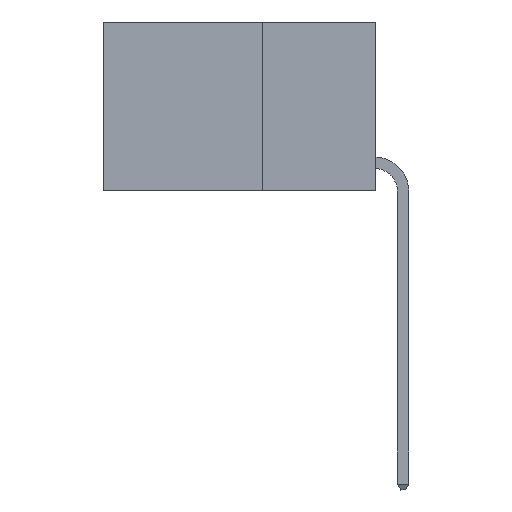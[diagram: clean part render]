
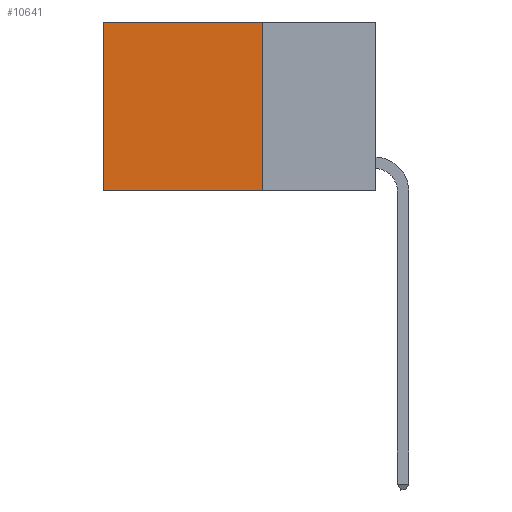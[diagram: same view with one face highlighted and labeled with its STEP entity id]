
A CAD part, left-side view. The second image highlights one B-rep face of the part: STEP entity #10641.
In plain terms, the highlighted planar face has unit normal (-1, 0, 0).
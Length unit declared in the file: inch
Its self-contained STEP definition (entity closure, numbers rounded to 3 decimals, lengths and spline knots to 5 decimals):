
#383 = ORIENTED_EDGE ( 'NONE', *, *, #12146, .T. ) ;
#412 = LINE ( 'NONE', #11326, #17715 ) ;
#622 = EDGE_CURVE ( 'NONE', #13639, #8643, #17457, .T. ) ;
#641 = CARTESIAN_POINT ( 'NONE',  ( 0.2625, 0.25, 0. ) ) ;
#673 = CARTESIAN_POINT ( 'NONE',  ( 0.2625, 0.6, 0. ) ) ;
#1697 = LINE ( 'NONE', #18123, #5662 ) ;
#2120 = DIRECTION ( 'NONE',  ( 0., 1., 0. ) ) ;
#2247 = DIRECTION ( 'NONE',  ( 0., 1., 0. ) ) ;
#3027 = VERTEX_POINT ( 'NONE', #14223 ) ;
#3090 = FACE_OUTER_BOUND ( 'NONE', #8799, .T. ) ;
#4413 = PLANE ( 'NONE',  #12980 ) ;
#5662 = VECTOR ( 'NONE', #7808, 39.37008 ) ;
#5687 = DIRECTION ( 'NONE',  ( 0., 0., -1. ) ) ;
#5933 = EDGE_CURVE ( 'NONE', #17601, #3027, #412, .T. ) ;
#6805 = LINE ( 'NONE', #673, #12048 ) ;
#7402 = CARTESIAN_POINT ( 'NONE',  ( 0.2625, 0.25, 0. ) ) ;
#7808 = DIRECTION ( 'NONE',  ( 0., 0., -1. ) ) ;
#8643 = VERTEX_POINT ( 'NONE', #17736 ) ;
#8799 = EDGE_LOOP ( 'NONE', ( #383, #10133, #10295, #11320 ) ) ;
#10133 = ORIENTED_EDGE ( 'NONE', *, *, #5933, .F. ) ;
#10295 = ORIENTED_EDGE ( 'NONE', *, *, #11871, .F. ) ;
#10506 = DIRECTION ( 'NONE',  ( 1., 0., 0. ) ) ;
#10641 = ADVANCED_FACE ( 'NONE', ( #3090 ), #4413, .F. ) ;
#11320 = ORIENTED_EDGE ( 'NONE', *, *, #622, .T. ) ;
#11326 = CARTESIAN_POINT ( 'NONE',  ( 0.2625, 0.25, -0.37 ) ) ;
#11871 = EDGE_CURVE ( 'NONE', #13639, #17601, #1697, .T. ) ;
#12048 = VECTOR ( 'NONE', #5687, 39.37008 ) ;
#12146 = EDGE_CURVE ( 'NONE', #8643, #3027, #6805, .T. ) ;
#12980 = AXIS2_PLACEMENT_3D ( 'NONE', #7402, #10506, #16530 ) ;
#13639 = VERTEX_POINT ( 'NONE', #19182 ) ;
#14223 = CARTESIAN_POINT ( 'NONE',  ( 0.2625, 0.6, -0.37 ) ) ;
#15623 = VECTOR ( 'NONE', #2247, 39.37008 ) ;
#16530 = DIRECTION ( 'NONE',  ( 0., 0., -1. ) ) ;
#17457 = LINE ( 'NONE', #641, #15623 ) ;
#17601 = VERTEX_POINT ( 'NONE', #18997 ) ;
#17715 = VECTOR ( 'NONE', #2120, 39.37008 ) ;
#17736 = CARTESIAN_POINT ( 'NONE',  ( 0.2625, 0.6, 0. ) ) ;
#18123 = CARTESIAN_POINT ( 'NONE',  ( 0.2625, 0.25, 0. ) ) ;
#18997 = CARTESIAN_POINT ( 'NONE',  ( 0.2625, 0.25, -0.37 ) ) ;
#19182 = CARTESIAN_POINT ( 'NONE',  ( 0.2625, 0.25, 0. ) ) ;
